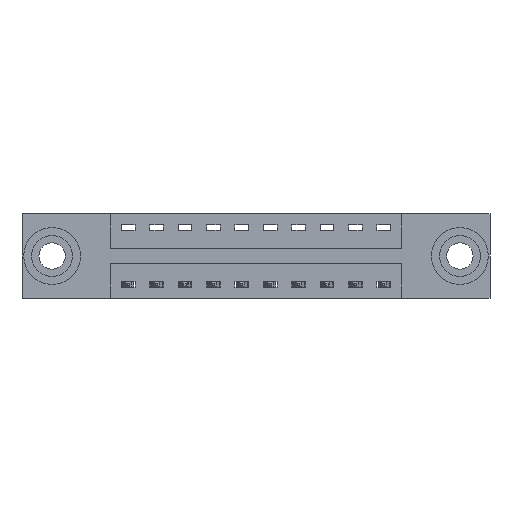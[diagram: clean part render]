
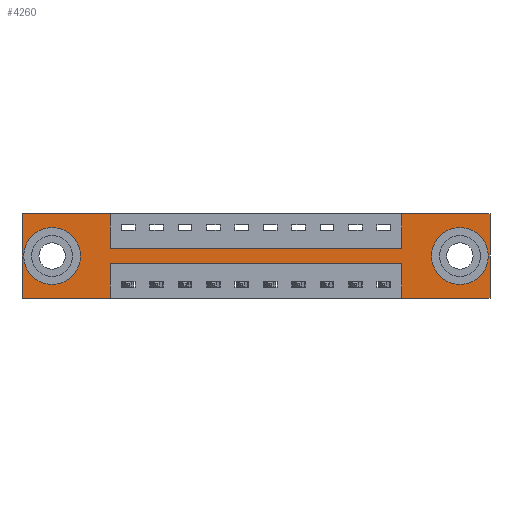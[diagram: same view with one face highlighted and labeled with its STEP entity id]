
A CAD part, front view. The second image highlights one B-rep face of the part: STEP entity #4260.
In plain terms, the highlighted planar face has unit normal (0, -1, 0).
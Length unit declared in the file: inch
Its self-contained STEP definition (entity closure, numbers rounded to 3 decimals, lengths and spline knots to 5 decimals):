
#1 = LINE ( 'NONE', #4904, #543 ) ;
#3 = CARTESIAN_POINT ( 'NONE',  ( 0., 0., 0. ) ) ;
#92 = VECTOR ( 'NONE', #3534, 39.37008 ) ;
#152 = CARTESIAN_POINT ( 'NONE',  ( 0.1325, 0., -0.263 ) ) ;
#187 = LINE ( 'NONE', #8529, #10214 ) ;
#222 = VERTEX_POINT ( 'NONE', #1277 ) ;
#307 = VERTEX_POINT ( 'NONE', #7367 ) ;
#504 = EDGE_CURVE ( 'NONE', #8015, #3206, #2114, .T. ) ;
#543 = VECTOR ( 'NONE', #6602, 39.37008 ) ;
#573 = CARTESIAN_POINT ( 'NONE',  ( 0.1325, 0., -0.185 ) ) ;
#610 = VERTEX_POINT ( 'NONE', #152 ) ;
#647 = EDGE_CURVE ( 'NONE', #7882, #6054, #1571, .T. ) ;
#795 = CARTESIAN_POINT ( 'NONE',  ( 0.3875, 0., 0. ) ) ;
#804 = ORIENTED_EDGE ( 'NONE', *, *, #10760, .T. ) ;
#820 = CARTESIAN_POINT ( 'NONE',  ( 0., 0., -0.37 ) ) ;
#861 = ORIENTED_EDGE ( 'NONE', *, *, #7101, .F. ) ;
#980 = CARTESIAN_POINT ( 'NONE',  ( 1.6725, 0., -0.22 ) ) ;
#1245 = VERTEX_POINT ( 'NONE', #10255 ) ;
#1277 = CARTESIAN_POINT ( 'NONE',  ( 0., 0., 0. ) ) ;
#1506 = EDGE_CURVE ( 'NONE', #8894, #610, #9470, .T. ) ;
#1515 = ORIENTED_EDGE ( 'NONE', *, *, #5993, .F. ) ;
#1543 = CARTESIAN_POINT ( 'NONE',  ( 0., 0., -0.37 ) ) ;
#1547 = DIRECTION ( 'NONE',  ( 1., 0., 0. ) ) ;
#1563 = DIRECTION ( 'NONE',  ( 1., 0., 0. ) ) ;
#1571 = LINE ( 'NONE', #7810, #11132 ) ;
#1708 = CARTESIAN_POINT ( 'NONE',  ( 1.6725, 0., 0. ) ) ;
#1823 = VECTOR ( 'NONE', #5959, 39.37008 ) ;
#1952 = ORIENTED_EDGE ( 'NONE', *, *, #6062, .F. ) ;
#2074 = LINE ( 'NONE', #7834, #5879 ) ;
#2114 = LINE ( 'NONE', #4190, #6196 ) ;
#2177 = ORIENTED_EDGE ( 'NONE', *, *, #647, .F. ) ;
#2181 = DIRECTION ( 'NONE',  ( 0., 1., 0. ) ) ;
#2227 = DIRECTION ( 'NONE',  ( 0., 0., -1. ) ) ;
#2353 = CARTESIAN_POINT ( 'NONE',  ( 1.6725, 0., -0.37 ) ) ;
#2360 = ORIENTED_EDGE ( 'NONE', *, *, #504, .F. ) ;
#2550 = EDGE_CURVE ( 'NONE', #3206, #4270, #6053, .T. ) ;
#2577 = CARTESIAN_POINT ( 'NONE',  ( 0.1325, 0., -0.107 ) ) ;
#2650 = VECTOR ( 'NONE', #4833, 39.37008 ) ;
#2673 = CIRCLE ( 'NONE', #3871, 0.078 ) ;
#2679 = DIRECTION ( 'NONE',  ( 0., -1., 0. ) ) ;
#2708 = LINE ( 'NONE', #795, #4334 ) ;
#2739 = EDGE_CURVE ( 'NONE', #4270, #7882, #187, .T. ) ;
#2878 = AXIS2_PLACEMENT_3D ( 'NONE', #7454, #2181, #8251 ) ;
#3146 = EDGE_CURVE ( 'NONE', #6054, #7592, #3947, .T. ) ;
#3148 = AXIS2_PLACEMENT_3D ( 'NONE', #573, #6709, #4941 ) ;
#3206 = VERTEX_POINT ( 'NONE', #2353 ) ;
#3233 = ORIENTED_EDGE ( 'NONE', *, *, #8925, .F. ) ;
#3534 = DIRECTION ( 'NONE',  ( 1., 0., 0. ) ) ;
#3577 = DIRECTION ( 'NONE',  ( -1., 0., 0. ) ) ;
#3688 = VERTEX_POINT ( 'NONE', #1708 ) ;
#3818 = DIRECTION ( 'NONE',  ( 0., 1., 0. ) ) ;
#3849 = LINE ( 'NONE', #4998, #1823 ) ;
#3852 = FACE_BOUND ( 'NONE', #8695, .T. ) ;
#3871 = AXIS2_PLACEMENT_3D ( 'NONE', #3939, #4805, #2227 ) ;
#3939 = CARTESIAN_POINT ( 'NONE',  ( 1.9275, 0., -0.185 ) ) ;
#3947 = LINE ( 'NONE', #1543, #5998 ) ;
#4006 = CARTESIAN_POINT ( 'NONE',  ( 1.6725, 0., -0.37 ) ) ;
#4190 = CARTESIAN_POINT ( 'NONE',  ( 0., 0., -0.37 ) ) ;
#4260 = ADVANCED_FACE ( 'NONE', ( #6306, #3852, #5903 ), #6962, .T. ) ;
#4270 = VERTEX_POINT ( 'NONE', #980 ) ;
#4281 = DIRECTION ( 'NONE',  ( 0., 0., -1. ) ) ;
#4334 = VECTOR ( 'NONE', #4281, 39.37008 ) ;
#4506 = VECTOR ( 'NONE', #9086, 39.37008 ) ;
#4805 = DIRECTION ( 'NONE',  ( 0., 1., 0. ) ) ;
#4833 = DIRECTION ( 'NONE',  ( 0., 0., 1. ) ) ;
#4904 = CARTESIAN_POINT ( 'NONE',  ( 1.6725, 0., 0. ) ) ;
#4941 = DIRECTION ( 'NONE',  ( 0., 0., 1. ) ) ;
#4988 = VERTEX_POINT ( 'NONE', #8644 ) ;
#4998 = CARTESIAN_POINT ( 'NONE',  ( 2.06, 0., 0. ) ) ;
#5036 = CARTESIAN_POINT ( 'NONE',  ( 0.3875, 0., -0.37 ) ) ;
#5069 = ORIENTED_EDGE ( 'NONE', *, *, #1506, .T. ) ;
#5103 = CARTESIAN_POINT ( 'NONE',  ( 0.3875, 0., -0.22 ) ) ;
#5170 = CIRCLE ( 'NONE', #2878, 0.078 ) ;
#5290 = VERTEX_POINT ( 'NONE', #9835 ) ;
#5375 = CARTESIAN_POINT ( 'NONE',  ( 0.3875, 0., -0.15 ) ) ;
#5668 = EDGE_LOOP ( 'NONE', ( #10797, #7649 ) ) ;
#5772 = CARTESIAN_POINT ( 'NONE',  ( 0., 0., 0. ) ) ;
#5800 = ORIENTED_EDGE ( 'NONE', *, *, #2550, .F. ) ;
#5879 = VECTOR ( 'NONE', #1563, 39.37008 ) ;
#5903 = FACE_OUTER_BOUND ( 'NONE', #6900, .T. ) ;
#5959 = DIRECTION ( 'NONE',  ( 0., 0., -1. ) ) ;
#5993 = EDGE_CURVE ( 'NONE', #7592, #222, #8166, .T. ) ;
#5998 = VECTOR ( 'NONE', #9281, 39.37008 ) ;
#6053 = LINE ( 'NONE', #4006, #2650 ) ;
#6054 = VERTEX_POINT ( 'NONE', #5036 ) ;
#6062 = EDGE_CURVE ( 'NONE', #10252, #8015, #3849, .T. ) ;
#6085 = VECTOR ( 'NONE', #1547, 39.37008 ) ;
#6196 = VECTOR ( 'NONE', #10372, 39.37008 ) ;
#6306 = FACE_BOUND ( 'NONE', #5668, .T. ) ;
#6393 = AXIS2_PLACEMENT_3D ( 'NONE', #820, #2679, #9538 ) ;
#6602 = DIRECTION ( 'NONE',  ( 0., 0., 1. ) ) ;
#6709 = DIRECTION ( 'NONE',  ( 0., 1., 0. ) ) ;
#6862 = ORIENTED_EDGE ( 'NONE', *, *, #11151, .F. ) ;
#6900 = EDGE_LOOP ( 'NONE', ( #2177, #8946, #5800, #2360, #1952, #861, #7693, #6862, #3233, #10111, #1515, #9108 ) ) ;
#6962 = PLANE ( 'NONE',  #6393 ) ;
#7101 = EDGE_CURVE ( 'NONE', #3688, #10252, #2074, .T. ) ;
#7367 = CARTESIAN_POINT ( 'NONE',  ( 1.9275, 0., -0.263 ) ) ;
#7454 = CARTESIAN_POINT ( 'NONE',  ( 1.9275, 0., -0.185 ) ) ;
#7592 = VERTEX_POINT ( 'NONE', #7678 ) ;
#7649 = ORIENTED_EDGE ( 'NONE', *, *, #10436, .T. ) ;
#7678 = CARTESIAN_POINT ( 'NONE',  ( 0., 0., -0.37 ) ) ;
#7693 = ORIENTED_EDGE ( 'NONE', *, *, #7825, .F. ) ;
#7742 = EDGE_CURVE ( 'NONE', #1245, #307, #5170, .T. ) ;
#7810 = CARTESIAN_POINT ( 'NONE',  ( 0.3875, 0., -0.37 ) ) ;
#7825 = EDGE_CURVE ( 'NONE', #5290, #3688, #1, .T. ) ;
#7834 = CARTESIAN_POINT ( 'NONE',  ( 0., 0., 0. ) ) ;
#7882 = VERTEX_POINT ( 'NONE', #5103 ) ;
#8015 = VERTEX_POINT ( 'NONE', #8604 ) ;
#8166 = LINE ( 'NONE', #5772, #4506 ) ;
#8176 = DIRECTION ( 'NONE',  ( 0., 0., 1. ) ) ;
#8251 = DIRECTION ( 'NONE',  ( 0., 0., -1. ) ) ;
#8529 = CARTESIAN_POINT ( 'NONE',  ( 0.3875, 0., -0.22 ) ) ;
#8604 = CARTESIAN_POINT ( 'NONE',  ( 2.06, 0., -0.37 ) ) ;
#8622 = LINE ( 'NONE', #3, #92 ) ;
#8644 = CARTESIAN_POINT ( 'NONE',  ( 0.3875, 0., 0. ) ) ;
#8695 = EDGE_LOOP ( 'NONE', ( #5069, #804 ) ) ;
#8752 = DIRECTION ( 'NONE',  ( 0., 0., -1. ) ) ;
#8894 = VERTEX_POINT ( 'NONE', #2577 ) ;
#8925 = EDGE_CURVE ( 'NONE', #4988, #10208, #2708, .T. ) ;
#8946 = ORIENTED_EDGE ( 'NONE', *, *, #2739, .F. ) ;
#9086 = DIRECTION ( 'NONE',  ( 0., 0., 1. ) ) ;
#9108 = ORIENTED_EDGE ( 'NONE', *, *, #3146, .F. ) ;
#9281 = DIRECTION ( 'NONE',  ( -1., 0., 0. ) ) ;
#9470 = CIRCLE ( 'NONE', #9908, 0.078 ) ;
#9538 = DIRECTION ( 'NONE',  ( 0., 0., -1. ) ) ;
#9786 = CARTESIAN_POINT ( 'NONE',  ( 2.06, 0., 0. ) ) ;
#9835 = CARTESIAN_POINT ( 'NONE',  ( 1.6725, 0., -0.15 ) ) ;
#9908 = AXIS2_PLACEMENT_3D ( 'NONE', #10725, #3818, #8176 ) ;
#10093 = CIRCLE ( 'NONE', #3148, 0.078 ) ;
#10111 = ORIENTED_EDGE ( 'NONE', *, *, #10958, .F. ) ;
#10208 = VERTEX_POINT ( 'NONE', #5375 ) ;
#10214 = VECTOR ( 'NONE', #3577, 39.37008 ) ;
#10252 = VERTEX_POINT ( 'NONE', #9786 ) ;
#10255 = CARTESIAN_POINT ( 'NONE',  ( 1.9275, 0., -0.107 ) ) ;
#10372 = DIRECTION ( 'NONE',  ( -1., 0., 0. ) ) ;
#10436 = EDGE_CURVE ( 'NONE', #307, #1245, #2673, .T. ) ;
#10649 = LINE ( 'NONE', #10781, #6085 ) ;
#10725 = CARTESIAN_POINT ( 'NONE',  ( 0.1325, 0., -0.185 ) ) ;
#10760 = EDGE_CURVE ( 'NONE', #610, #8894, #10093, .T. ) ;
#10781 = CARTESIAN_POINT ( 'NONE',  ( 0.3875, 0., -0.15 ) ) ;
#10797 = ORIENTED_EDGE ( 'NONE', *, *, #7742, .T. ) ;
#10958 = EDGE_CURVE ( 'NONE', #222, #4988, #8622, .T. ) ;
#11132 = VECTOR ( 'NONE', #8752, 39.37008 ) ;
#11151 = EDGE_CURVE ( 'NONE', #10208, #5290, #10649, .T. ) ;
